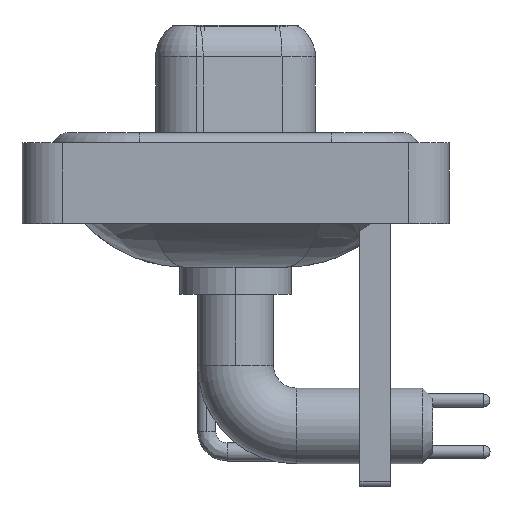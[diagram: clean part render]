
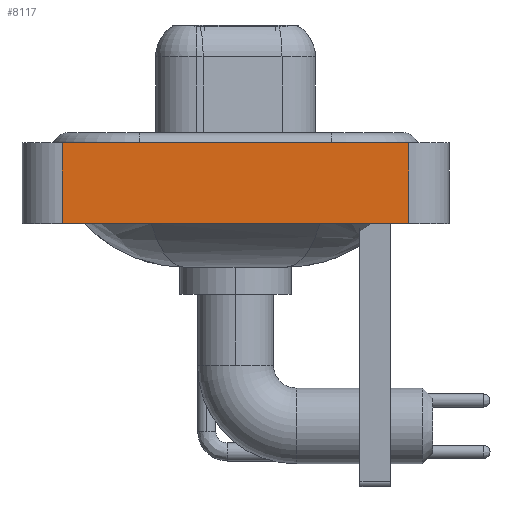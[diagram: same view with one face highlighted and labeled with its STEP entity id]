
A CAD part, left-side view. The second image highlights one B-rep face of the part: STEP entity #8117.
In plain terms, the highlighted planar face has unit normal (-1, 0, 0).
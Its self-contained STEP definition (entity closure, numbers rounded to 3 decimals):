
#586 = CARTESIAN_POINT ( 'NONE',  ( -7.35, 8.55, 0.4 ) ) ;
#880 = VERTEX_POINT ( 'NONE', #17299 ) ;
#1119 = LINE ( 'NONE', #20856, #13782 ) ;
#1321 = FACE_OUTER_BOUND ( 'NONE', #10951, .T. ) ;
#1342 = LINE ( 'NONE', #13345, #21251 ) ;
#2312 = ORIENTED_EDGE ( 'NONE', *, *, #12054, .F. ) ;
#2374 = CARTESIAN_POINT ( 'NONE',  ( -7.35, 8.55, -3.6 ) ) ;
#2502 = LINE ( 'NONE', #2727, #5379 ) ;
#2727 = CARTESIAN_POINT ( 'NONE',  ( -7.35, -8.55, -3.6 ) ) ;
#2836 = DIRECTION ( 'NONE',  ( 0., 0., 1. ) ) ;
#2868 = DIRECTION ( 'NONE',  ( 0., 0., 1. ) ) ;
#2883 = DIRECTION ( 'NONE',  ( 0., -1., 0. ) ) ;
#4689 = ORIENTED_EDGE ( 'NONE', *, *, #13364, .T. ) ;
#5379 = VECTOR ( 'NONE', #14626, 1000. ) ;
#5961 = VERTEX_POINT ( 'NONE', #586 ) ;
#6011 = VERTEX_POINT ( 'NONE', #20331 ) ;
#6676 = ORIENTED_EDGE ( 'NONE', *, *, #15467, .F. ) ;
#8117 = ADVANCED_FACE ( 'NONE', ( #1321 ), #19957, .T. ) ;
#8802 = VERTEX_POINT ( 'NONE', #2374 ) ;
#10951 = EDGE_LOOP ( 'NONE', ( #4689, #2312, #6676, #17077 ) ) ;
#10976 = AXIS2_PLACEMENT_3D ( 'NONE', #17965, #19840, #2868 ) ;
#11203 = CARTESIAN_POINT ( 'NONE',  ( -7.35, 8.55, -3.6 ) ) ;
#12054 = EDGE_CURVE ( 'NONE', #5961, #880, #1119, .T. ) ;
#13345 = CARTESIAN_POINT ( 'NONE',  ( -7.35, -8.55, -3.6 ) ) ;
#13364 = EDGE_CURVE ( 'NONE', #6011, #880, #1342, .T. ) ;
#13782 = VECTOR ( 'NONE', #2883, 1000. ) ;
#14626 = DIRECTION ( 'NONE',  ( 0., -1., 0. ) ) ;
#15426 = EDGE_CURVE ( 'NONE', #8802, #6011, #2502, .T. ) ;
#15467 = EDGE_CURVE ( 'NONE', #8802, #5961, #19155, .T. ) ;
#17077 = ORIENTED_EDGE ( 'NONE', *, *, #15426, .T. ) ;
#17299 = CARTESIAN_POINT ( 'NONE',  ( -7.35, -8.55, 0.4 ) ) ;
#17686 = VECTOR ( 'NONE', #2836, 1000. ) ;
#17965 = CARTESIAN_POINT ( 'NONE',  ( -7.35, -8.55, -3.6 ) ) ;
#18202 = DIRECTION ( 'NONE',  ( 0., 0., 1. ) ) ;
#19155 = LINE ( 'NONE', #11203, #17686 ) ;
#19840 = DIRECTION ( 'NONE',  ( -1., 0., 0. ) ) ;
#19957 = PLANE ( 'NONE',  #10976 ) ;
#20331 = CARTESIAN_POINT ( 'NONE',  ( -7.35, -8.55, -3.6 ) ) ;
#20856 = CARTESIAN_POINT ( 'NONE',  ( -7.35, -8.55, 0.4 ) ) ;
#21251 = VECTOR ( 'NONE', #18202, 1000. ) ;
